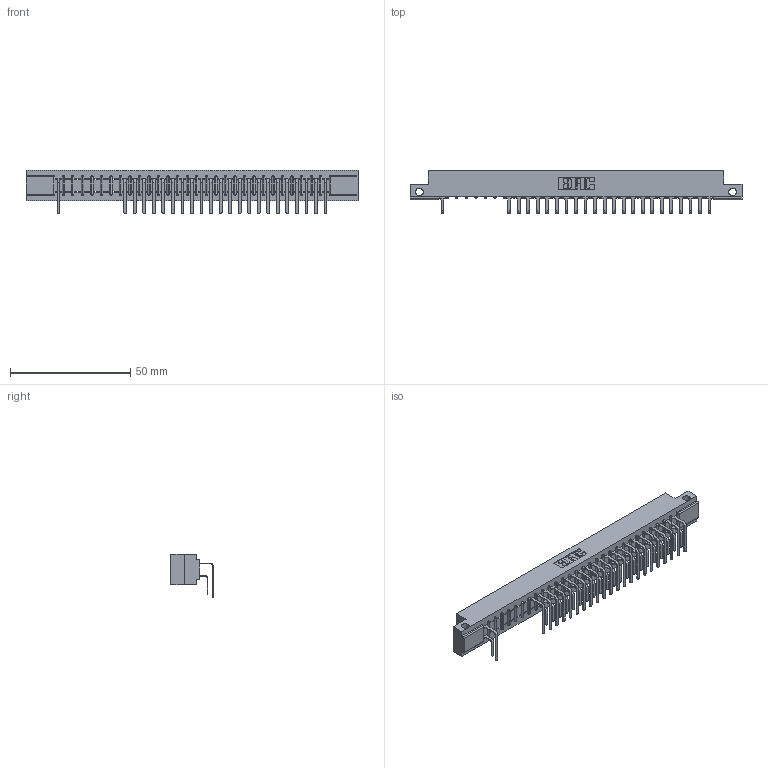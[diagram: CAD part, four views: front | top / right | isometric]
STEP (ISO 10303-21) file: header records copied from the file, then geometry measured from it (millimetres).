
FILE_DESCRIPTION (( 'STEP AP203' ), '1' );
FILE_NAME ('357-029-559-112.STEP', '2018-08-09T07:52:34', ( '' ), ( '' ), 'SwSTEP 2.0', 'SolidWorks 2016', '' );
FILE_SCHEMA (( 'CONFIG_CONTROL_DESIGN' ));
Length unit declared in the file: inch
Products named in the file (4): 307 Part_.128 Dia Side Mounting Holes; 307-290-001_558 559 - 1 (Single); 307-290-001_559 - 2 (Single); 357-029-559-112
Assembly tree (46 placements, depth 2):
  357-029-559-112
    307 Part_.128 Dia Side Mounting Holes
    307-290-001_558 559 - 1 (Single)  x22
    307-290-001_559 - 2 (Single)  x23
Bounding box: 137.92 x 17.69 x 18.07 mm (x, y, z)
Volume: 14465 mm3; surface area: 17489.6 mm2
Topology: 46 solids, 46 shells, 2528 faces, 7129 edges, 4610 vertices
Faces by surface type: plane 1633, cylinder 835, sphere 60
Entity records: 28425 total; most frequent: CARTESIAN_POINT 4710, ORIENTED_EDGE 4678, DIRECTION 4605, EDGE_CURVE 2339, LINE 1787, VECTOR 1787, VERTEX_POINT 1514, AXIS2_PLACEMENT_3D 1409
